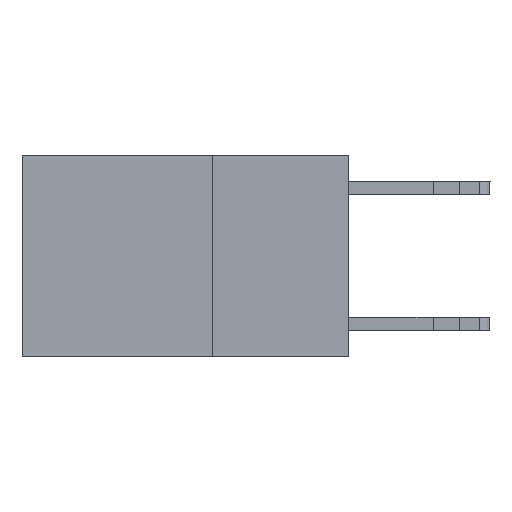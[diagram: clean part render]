
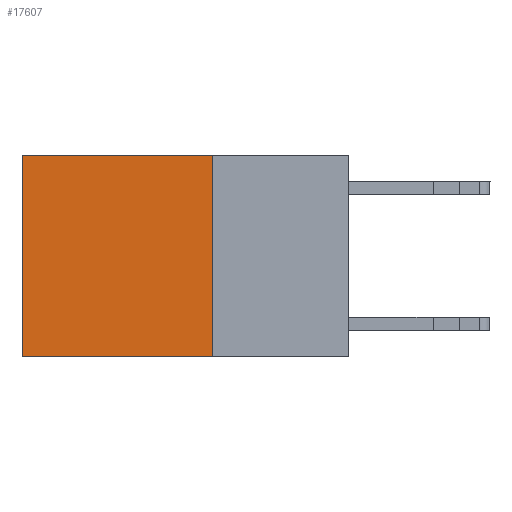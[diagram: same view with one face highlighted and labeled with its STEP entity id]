
A CAD part, left-side view. The second image highlights one B-rep face of the part: STEP entity #17607.
In plain terms, the highlighted planar face has unit normal (-1, 0, 0).
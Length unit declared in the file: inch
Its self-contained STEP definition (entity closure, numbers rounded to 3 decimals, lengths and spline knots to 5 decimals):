
#6 = ORIENTED_EDGE ( 'NONE', *, *, #2842, .T. ) ;
#330 = DIRECTION ( 'NONE',  ( 0., 0., -1. ) ) ;
#606 = CARTESIAN_POINT ( 'NONE',  ( 0.2625, 0.25, 0. ) ) ;
#1038 = DIRECTION ( 'NONE',  ( 0., 1., 0. ) ) ;
#1904 = CARTESIAN_POINT ( 'NONE',  ( 0.2625, 0.25, 0. ) ) ;
#2188 = PLANE ( 'NONE',  #17791 ) ;
#2612 = ORIENTED_EDGE ( 'NONE', *, *, #3768, .F. ) ;
#2776 = CARTESIAN_POINT ( 'NONE',  ( 0.2625, 0.25, -0.37 ) ) ;
#2842 = EDGE_CURVE ( 'NONE', #14056, #19627, #21374, .T. ) ;
#3016 = VECTOR ( 'NONE', #1038, 39.37008 ) ;
#3031 = LINE ( 'NONE', #2776, #3016 ) ;
#3768 = EDGE_CURVE ( 'NONE', #22263, #5241, #3031, .T. ) ;
#5241 = VERTEX_POINT ( 'NONE', #22349 ) ;
#8530 = EDGE_CURVE ( 'NONE', #19627, #5241, #11531, .T. ) ;
#9012 = VECTOR ( 'NONE', #23206, 39.37008 ) ;
#9135 = CARTESIAN_POINT ( 'NONE',  ( 0.2625, 0.25, -0.37 ) ) ;
#9504 = EDGE_LOOP ( 'NONE', ( #25324, #2612, #25105, #6 ) ) ;
#9568 = VECTOR ( 'NONE', #330, 39.37008 ) ;
#11468 = CARTESIAN_POINT ( 'NONE',  ( 0.2625, 0.25, 0. ) ) ;
#11531 = LINE ( 'NONE', #14014, #9568 ) ;
#13551 = LINE ( 'NONE', #11468, #25059 ) ;
#14014 = CARTESIAN_POINT ( 'NONE',  ( 0.2625, 0.6, 0. ) ) ;
#14056 = VERTEX_POINT ( 'NONE', #1904 ) ;
#16643 = FACE_OUTER_BOUND ( 'NONE', #9504, .T. ) ;
#17607 = ADVANCED_FACE ( 'NONE', ( #16643 ), #2188, .F. ) ;
#17791 = AXIS2_PLACEMENT_3D ( 'NONE', #606, #18227, #18495 ) ;
#18227 = DIRECTION ( 'NONE',  ( 1., 0., 0. ) ) ;
#18495 = DIRECTION ( 'NONE',  ( 0., 0., -1. ) ) ;
#19627 = VERTEX_POINT ( 'NONE', #19847 ) ;
#19847 = CARTESIAN_POINT ( 'NONE',  ( 0.2625, 0.6, 0. ) ) ;
#21374 = LINE ( 'NONE', #22954, #9012 ) ;
#22263 = VERTEX_POINT ( 'NONE', #9135 ) ;
#22349 = CARTESIAN_POINT ( 'NONE',  ( 0.2625, 0.6, -0.37 ) ) ;
#22954 = CARTESIAN_POINT ( 'NONE',  ( 0.2625, 0.25, 0. ) ) ;
#23206 = DIRECTION ( 'NONE',  ( 0., 1., 0. ) ) ;
#24935 = EDGE_CURVE ( 'NONE', #14056, #22263, #13551, .T. ) ;
#25059 = VECTOR ( 'NONE', #25524, 39.37008 ) ;
#25105 = ORIENTED_EDGE ( 'NONE', *, *, #24935, .F. ) ;
#25324 = ORIENTED_EDGE ( 'NONE', *, *, #8530, .T. ) ;
#25524 = DIRECTION ( 'NONE',  ( 0., 0., -1. ) ) ;
